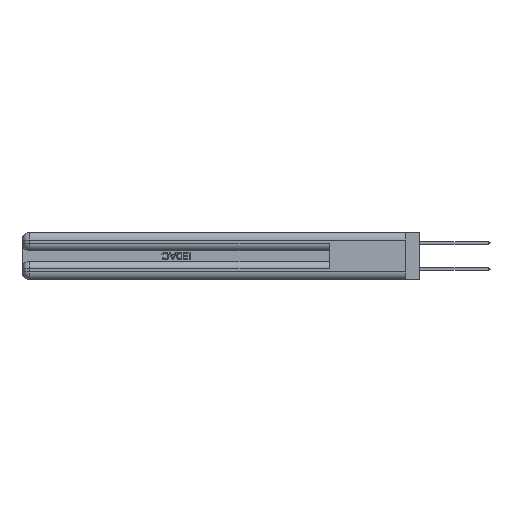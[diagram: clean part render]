
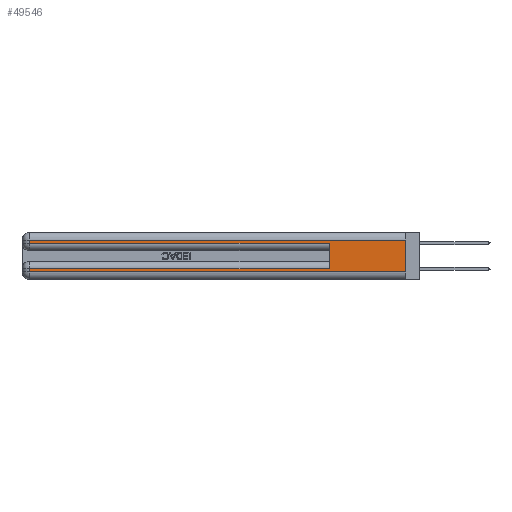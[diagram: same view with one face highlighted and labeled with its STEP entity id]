
A CAD part, left-side view. The second image highlights one B-rep face of the part: STEP entity #49546.
In plain terms, the highlighted planar face has unit normal (-1, 0, 0).
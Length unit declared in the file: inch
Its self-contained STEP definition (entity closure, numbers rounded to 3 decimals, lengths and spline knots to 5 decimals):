
#203 = CARTESIAN_POINT ( 'NONE',  ( 0., 0.6, 0.145 ) ) ;
#3041 = EDGE_CURVE ( 'NONE', #31723, #40501, #42525, .T. ) ;
#3655 = CARTESIAN_POINT ( 'NONE',  ( 0., 0.6, 0.085 ) ) ;
#4482 = ORIENTED_EDGE ( 'NONE', *, *, #24074, .T. ) ;
#4624 = LINE ( 'NONE', #47438, #44991 ) ;
#6207 = CARTESIAN_POINT ( 'NONE',  ( 0., 0., 0.37 ) ) ;
#6886 = ORIENTED_EDGE ( 'NONE', *, *, #48765, .T. ) ;
#7064 = VECTOR ( 'NONE', #25018, 39.37008 ) ;
#9046 = DIRECTION ( 'NONE',  ( 0., 1., 0. ) ) ;
#9285 = CARTESIAN_POINT ( 'NONE',  ( 0., 0., 0.37 ) ) ;
#9799 = EDGE_CURVE ( 'NONE', #39008, #15637, #24834, .T. ) ;
#10158 = DIRECTION ( 'NONE',  ( 0., 0., -1. ) ) ;
#10617 = ORIENTED_EDGE ( 'NONE', *, *, #31040, .T. ) ;
#11336 = CARTESIAN_POINT ( 'NONE',  ( 0., 0.6, 0.285 ) ) ;
#13032 = EDGE_CURVE ( 'NONE', #19216, #40381, #40062, .T. ) ;
#14426 = VECTOR ( 'NONE', #17113, 39.37008 ) ;
#15637 = VERTEX_POINT ( 'NONE', #50440 ) ;
#15881 = CARTESIAN_POINT ( 'NONE',  ( 0., 2.94, 0.06 ) ) ;
#16308 = DIRECTION ( 'NONE',  ( 0., 0., -1. ) ) ;
#16682 = CARTESIAN_POINT ( 'NONE',  ( 0., 0., 0.085 ) ) ;
#17113 = DIRECTION ( 'NONE',  ( 0., 0., -1. ) ) ;
#18163 = VECTOR ( 'NONE', #39319, 39.37008 ) ;
#19216 = VERTEX_POINT ( 'NONE', #23166 ) ;
#20165 = DIRECTION ( 'NONE',  ( 0., 1., 0. ) ) ;
#21807 = CARTESIAN_POINT ( 'NONE',  ( 0., 0., 0.285 ) ) ;
#23166 = CARTESIAN_POINT ( 'NONE',  ( 0., 2.94, 0.085 ) ) ;
#23228 = VECTOR ( 'NONE', #9046, 39.37008 ) ;
#23507 = EDGE_LOOP ( 'NONE', ( #25287, #4482, #39172, #44010, #39256, #6886, #44790, #10617 ) ) ;
#23882 = CARTESIAN_POINT ( 'NONE',  ( 0., 0., 0.31 ) ) ;
#24074 = EDGE_CURVE ( 'NONE', #39008, #31723, #4624, .T. ) ;
#24834 = LINE ( 'NONE', #9285, #14426 ) ;
#25018 = DIRECTION ( 'NONE',  ( 0., -1., 0. ) ) ;
#25287 = ORIENTED_EDGE ( 'NONE', *, *, #9799, .F. ) ;
#25710 = LINE ( 'NONE', #16682, #23228 ) ;
#26218 = DIRECTION ( 'NONE',  ( 0., 0., -1. ) ) ;
#28519 = VECTOR ( 'NONE', #16308, 39.37008 ) ;
#29876 = LINE ( 'NONE', #203, #18163 ) ;
#30153 = AXIS2_PLACEMENT_3D ( 'NONE', #6207, #33623, #10158 ) ;
#30273 = LINE ( 'NONE', #21807, #39372 ) ;
#31040 = EDGE_CURVE ( 'NONE', #40381, #15637, #47343, .T. ) ;
#31723 = VERTEX_POINT ( 'NONE', #33528 ) ;
#32886 = EDGE_CURVE ( 'NONE', #35290, #49786, #29876, .T. ) ;
#33440 = VECTOR ( 'NONE', #26218, 39.37008 ) ;
#33528 = CARTESIAN_POINT ( 'NONE',  ( 0., 2.94, 0.31 ) ) ;
#33623 = DIRECTION ( 'NONE',  ( 1., 0., 0. ) ) ;
#35290 = VERTEX_POINT ( 'NONE', #3655 ) ;
#36533 = CARTESIAN_POINT ( 'NONE',  ( 0., 2.94, 0.37 ) ) ;
#36823 = CARTESIAN_POINT ( 'NONE',  ( 0., 0., 0.06 ) ) ;
#36965 = CARTESIAN_POINT ( 'NONE',  ( 0., 2.94, 0.285 ) ) ;
#39008 = VERTEX_POINT ( 'NONE', #23882 ) ;
#39172 = ORIENTED_EDGE ( 'NONE', *, *, #3041, .T. ) ;
#39256 = ORIENTED_EDGE ( 'NONE', *, *, #32886, .F. ) ;
#39319 = DIRECTION ( 'NONE',  ( 0., 0., 1. ) ) ;
#39372 = VECTOR ( 'NONE', #45112, 39.37008 ) ;
#40062 = LINE ( 'NONE', #36533, #28519 ) ;
#40381 = VERTEX_POINT ( 'NONE', #15881 ) ;
#40501 = VERTEX_POINT ( 'NONE', #36965 ) ;
#42525 = LINE ( 'NONE', #49461, #33440 ) ;
#44010 = ORIENTED_EDGE ( 'NONE', *, *, #45436, .T. ) ;
#44790 = ORIENTED_EDGE ( 'NONE', *, *, #13032, .T. ) ;
#44991 = VECTOR ( 'NONE', #20165, 39.37008 ) ;
#45112 = DIRECTION ( 'NONE',  ( 0., -1., 0. ) ) ;
#45436 = EDGE_CURVE ( 'NONE', #40501, #49786, #30273, .T. ) ;
#47343 = LINE ( 'NONE', #36823, #7064 ) ;
#47438 = CARTESIAN_POINT ( 'NONE',  ( 0., 0., 0.31 ) ) ;
#47492 = FACE_OUTER_BOUND ( 'NONE', #23507, .T. ) ;
#48765 = EDGE_CURVE ( 'NONE', #35290, #19216, #25710, .T. ) ;
#49023 = PLANE ( 'NONE',  #30153 ) ;
#49461 = CARTESIAN_POINT ( 'NONE',  ( 0., 2.94, 0.37 ) ) ;
#49546 = ADVANCED_FACE ( 'NONE', ( #47492 ), #49023, .F. ) ;
#49786 = VERTEX_POINT ( 'NONE', #11336 ) ;
#50440 = CARTESIAN_POINT ( 'NONE',  ( 0., 0., 0.06 ) ) ;
